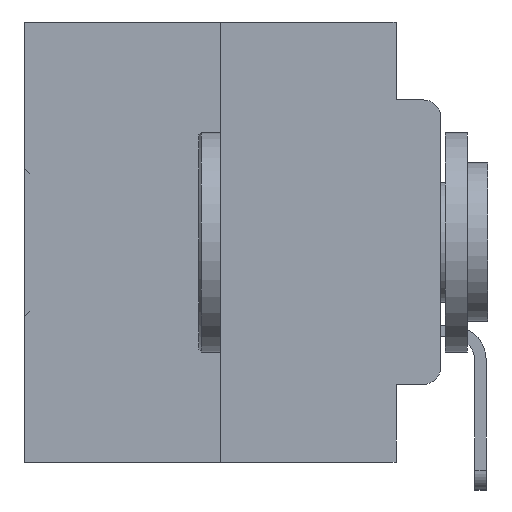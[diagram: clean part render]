
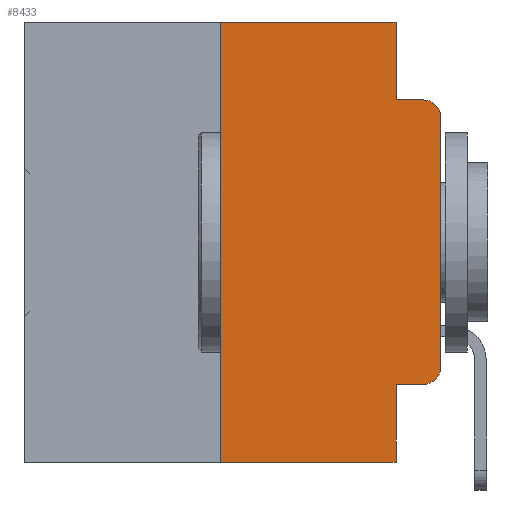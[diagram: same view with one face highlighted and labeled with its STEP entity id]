
A CAD part, left-side view. The second image highlights one B-rep face of the part: STEP entity #8433.
In plain terms, the highlighted planar face has unit normal (-1, 0, 0).
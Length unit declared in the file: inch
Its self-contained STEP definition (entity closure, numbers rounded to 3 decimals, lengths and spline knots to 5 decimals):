
#396 = DIRECTION ( 'NONE',  ( 0., 0., -1. ) ) ;
#430 = VECTOR ( 'NONE', #6106, 39.37008 ) ;
#577 = CARTESIAN_POINT ( 'NONE',  ( 0., 0.25, -0.5 ) ) ;
#615 = VERTEX_POINT ( 'NONE', #577 ) ;
#1546 = EDGE_CURVE ( 'NONE', #2959, #23135, #9324, .T. ) ;
#1807 = ORIENTED_EDGE ( 'NONE', *, *, #5445, .T. ) ;
#1992 = VECTOR ( 'NONE', #396, 39.37008 ) ;
#2016 = CARTESIAN_POINT ( 'NONE',  ( 0., 0.02, -0.0885 ) ) ;
#2127 = CARTESIAN_POINT ( 'NONE',  ( 0., 0.25, 0. ) ) ;
#2567 = EDGE_CURVE ( 'NONE', #33506, #8488, #13232, .T. ) ;
#2742 = ORIENTED_EDGE ( 'NONE', *, *, #2567, .F. ) ;
#2959 = VERTEX_POINT ( 'NONE', #33205 ) ;
#4692 = VERTEX_POINT ( 'NONE', #19947 ) ;
#4708 = VERTEX_POINT ( 'NONE', #6342 ) ;
#5407 = ORIENTED_EDGE ( 'NONE', *, *, #30064, .F. ) ;
#5445 = EDGE_CURVE ( 'NONE', #22557, #8488, #27566, .T. ) ;
#6106 = DIRECTION ( 'NONE',  ( 0., -1., 0. ) ) ;
#6291 = ORIENTED_EDGE ( 'NONE', *, *, #1546, .F. ) ;
#6342 = CARTESIAN_POINT ( 'NONE',  ( 0., 0.051, 0. ) ) ;
#6543 = CARTESIAN_POINT ( 'NONE',  ( 0., 0.473, 0. ) ) ;
#6896 = CARTESIAN_POINT ( 'NONE',  ( 0., 0.473, -0.5 ) ) ;
#7154 = VERTEX_POINT ( 'NONE', #22683 ) ;
#7159 = FACE_OUTER_BOUND ( 'NONE', #13395, .T. ) ;
#7387 = DIRECTION ( 'NONE',  ( -1., 0., 0. ) ) ;
#8066 = ORIENTED_EDGE ( 'NONE', *, *, #8682, .T. ) ;
#8433 = ADVANCED_FACE ( 'NONE', ( #7159 ), #20888, .F. ) ;
#8432 = EDGE_CURVE ( 'NONE', #16453, #4692, #27379, .T. ) ;
#8488 = VERTEX_POINT ( 'NONE', #2016 ) ;
#8682 = EDGE_CURVE ( 'NONE', #2959, #16453, #21505, .T. ) ;
#8851 = EDGE_CURVE ( 'NONE', #7154, #4708, #17512, .T. ) ;
#9023 = DIRECTION ( 'NONE',  ( 0., 0., 1. ) ) ;
#9324 = LINE ( 'NONE', #26353, #15855 ) ;
#9380 = DIRECTION ( 'NONE',  ( 0., -1., 0. ) ) ;
#10214 = DIRECTION ( 'NONE',  ( 1., 0., 0. ) ) ;
#10254 = AXIS2_PLACEMENT_3D ( 'NONE', #31425, #16456, #33807 ) ;
#11609 = EDGE_CURVE ( 'NONE', #615, #23135, #16443, .T. ) ;
#12075 = CARTESIAN_POINT ( 'NONE',  ( 0., 0.02, -0.4115 ) ) ;
#13232 = LINE ( 'NONE', #16276, #26169 ) ;
#13395 = EDGE_LOOP ( 'NONE', ( #21926, #1807, #2742, #31590, #19157, #5407, #26618, #6291, #8066, #28961 ) ) ;
#13493 = DIRECTION ( 'NONE',  ( 0., -1., 0. ) ) ;
#14476 = CARTESIAN_POINT ( 'NONE',  ( 0., 0.051, 0. ) ) ;
#15855 = VECTOR ( 'NONE', #18879, 39.37008 ) ;
#16276 = CARTESIAN_POINT ( 'NONE',  ( 0., 0.051, -0.0885 ) ) ;
#16443 = LINE ( 'NONE', #6896, #29776 ) ;
#16453 = VERTEX_POINT ( 'NONE', #12075 ) ;
#16456 = DIRECTION ( 'NONE',  ( -1., 0., 0. ) ) ;
#16837 = AXIS2_PLACEMENT_3D ( 'NONE', #23426, #7387, #25936 ) ;
#16839 = LINE ( 'NONE', #22442, #22774 ) ;
#16918 = LINE ( 'NONE', #14476, #1992 ) ;
#17512 = LINE ( 'NONE', #6543, #28514 ) ;
#18167 = EDGE_CURVE ( 'NONE', #4708, #33506, #16918, .T. ) ;
#18879 = DIRECTION ( 'NONE',  ( 0., 0., -1. ) ) ;
#19157 = ORIENTED_EDGE ( 'NONE', *, *, #8851, .F. ) ;
#19448 = EDGE_CURVE ( 'NONE', #4692, #22557, #16839, .T. ) ;
#19947 = CARTESIAN_POINT ( 'NONE',  ( 0., 0., -0.3915 ) ) ;
#20888 = PLANE ( 'NONE',  #23640 ) ;
#21302 = DIRECTION ( 'NONE',  ( 0., 0., 1. ) ) ;
#21505 = LINE ( 'NONE', #24817, #430 ) ;
#21926 = ORIENTED_EDGE ( 'NONE', *, *, #19448, .T. ) ;
#22213 = CARTESIAN_POINT ( 'NONE',  ( 0., 0.051, -0.0885 ) ) ;
#22442 = CARTESIAN_POINT ( 'NONE',  ( 0., 0., 0. ) ) ;
#22557 = VERTEX_POINT ( 'NONE', #22706 ) ;
#22683 = CARTESIAN_POINT ( 'NONE',  ( 0., 0.25, 0. ) ) ;
#22706 = CARTESIAN_POINT ( 'NONE',  ( 0., 0., -0.1085 ) ) ;
#22774 = VECTOR ( 'NONE', #9023, 39.37008 ) ;
#23135 = VERTEX_POINT ( 'NONE', #30688 ) ;
#23426 = CARTESIAN_POINT ( 'NONE',  ( 0., 0.02, -0.3915 ) ) ;
#23640 = AXIS2_PLACEMENT_3D ( 'NONE', #30780, #10214, #28421 ) ;
#24709 = LINE ( 'NONE', #2127, #29704 ) ;
#24817 = CARTESIAN_POINT ( 'NONE',  ( 0., 0.051, -0.4115 ) ) ;
#25489 = DIRECTION ( 'NONE',  ( 0., -1., 0. ) ) ;
#25936 = DIRECTION ( 'NONE',  ( 0., 0., -1. ) ) ;
#26169 = VECTOR ( 'NONE', #13493, 39.37008 ) ;
#26353 = CARTESIAN_POINT ( 'NONE',  ( 0., 0.051, 0. ) ) ;
#26618 = ORIENTED_EDGE ( 'NONE', *, *, #11609, .T. ) ;
#27379 = CIRCLE ( 'NONE', #16837, 0.02 ) ;
#27566 = CIRCLE ( 'NONE', #10254, 0.02 ) ;
#28421 = DIRECTION ( 'NONE',  ( 0., 0., -1. ) ) ;
#28514 = VECTOR ( 'NONE', #9380, 39.37008 ) ;
#28961 = ORIENTED_EDGE ( 'NONE', *, *, #8432, .T. ) ;
#29704 = VECTOR ( 'NONE', #21302, 39.37008 ) ;
#29776 = VECTOR ( 'NONE', #25489, 39.37008 ) ;
#30064 = EDGE_CURVE ( 'NONE', #615, #7154, #24709, .T. ) ;
#30688 = CARTESIAN_POINT ( 'NONE',  ( 0., 0.051, -0.5 ) ) ;
#30780 = CARTESIAN_POINT ( 'NONE',  ( 0., 0.473, 0. ) ) ;
#31425 = CARTESIAN_POINT ( 'NONE',  ( 0., 0.02, -0.1085 ) ) ;
#31590 = ORIENTED_EDGE ( 'NONE', *, *, #18167, .F. ) ;
#33205 = CARTESIAN_POINT ( 'NONE',  ( 0., 0.051, -0.4115 ) ) ;
#33506 = VERTEX_POINT ( 'NONE', #22213 ) ;
#33807 = DIRECTION ( 'NONE',  ( 0., 0., -1. ) ) ;
